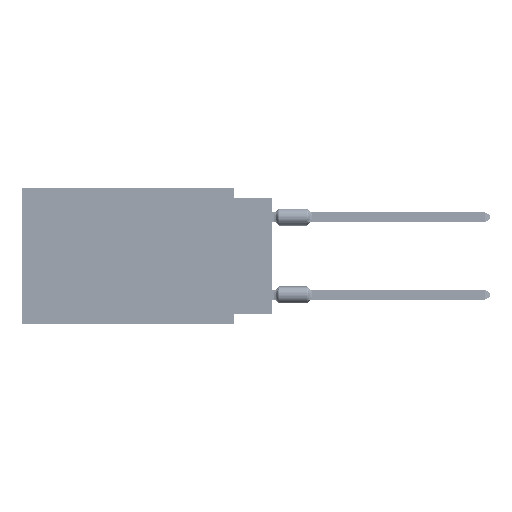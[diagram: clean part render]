
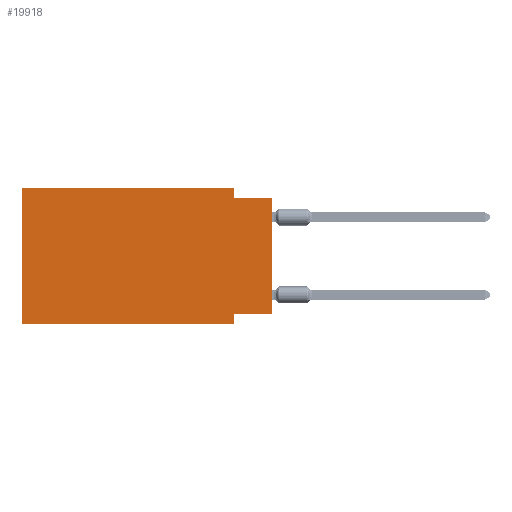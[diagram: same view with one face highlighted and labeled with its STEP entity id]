
A CAD part, left-side view. The second image highlights one B-rep face of the part: STEP entity #19918.
In plain terms, the highlighted planar face has unit normal (-1, 0, 0).
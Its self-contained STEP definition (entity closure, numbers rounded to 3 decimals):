
#172 = VERTEX_POINT ( 'NONE', #66391 ) ;
#1772 = LINE ( 'NONE', #67572, #3884 ) ;
#1815 = LINE ( 'NONE', #30420, #67050 ) ;
#2277 = DIRECTION ( 'NONE',  ( 0., 0., -1. ) ) ;
#2451 = EDGE_CURVE ( 'NONE', #49200, #65227, #50712, .T. ) ;
#3884 = VECTOR ( 'NONE', #35397, 1000. ) ;
#5882 = EDGE_CURVE ( 'NONE', #38103, #64522, #67398, .T. ) ;
#8389 = CARTESIAN_POINT ( 'NONE',  ( 0., 16.383, 0. ) ) ;
#10590 = DIRECTION ( 'NONE',  ( 0., -1., 0. ) ) ;
#10995 = DIRECTION ( 'NONE',  ( 0., 0., -1. ) ) ;
#12068 = EDGE_CURVE ( 'NONE', #49200, #19181, #1815, .T. ) ;
#12391 = FACE_OUTER_BOUND ( 'NONE', #24524, .T. ) ;
#12563 = CARTESIAN_POINT ( 'NONE',  ( 0., 2.54, -8.255 ) ) ;
#14311 = DIRECTION ( 'NONE',  ( 0., 1., 0. ) ) ;
#15615 = CARTESIAN_POINT ( 'NONE',  ( 0., 16.383, -8.89 ) ) ;
#16033 = AXIS2_PLACEMENT_3D ( 'NONE', #54968, #59996, #10995 ) ;
#16407 = CARTESIAN_POINT ( 'NONE',  ( 0., 0., -0.635 ) ) ;
#17709 = VECTOR ( 'NONE', #62150, 1000. ) ;
#18335 = DIRECTION ( 'NONE',  ( 0., 0., 1. ) ) ;
#18380 = CARTESIAN_POINT ( 'NONE',  ( 0., 2.54, 0. ) ) ;
#19181 = VERTEX_POINT ( 'NONE', #12563 ) ;
#19918 = ADVANCED_FACE ( 'NONE', ( #12391 ), #49604, .F. ) ;
#24398 = VERTEX_POINT ( 'NONE', #56808 ) ;
#24524 = EDGE_LOOP ( 'NONE', ( #34613, #55783, #64767, #27167, #53385, #25522, #66398, #43980 ) ) ;
#25398 = CARTESIAN_POINT ( 'NONE',  ( 0., 2.54, -8.89 ) ) ;
#25522 = ORIENTED_EDGE ( 'NONE', *, *, #68546, .T. ) ;
#27102 = EDGE_CURVE ( 'NONE', #172, #24398, #61634, .T. ) ;
#27167 = ORIENTED_EDGE ( 'NONE', *, *, #41906, .F. ) ;
#30194 = CARTESIAN_POINT ( 'NONE',  ( 0., 0., -0.635 ) ) ;
#30420 = CARTESIAN_POINT ( 'NONE',  ( 0., 0., -8.255 ) ) ;
#33171 = VECTOR ( 'NONE', #10590, 1000. ) ;
#33748 = CARTESIAN_POINT ( 'NONE',  ( 0., 2.54, -0.635 ) ) ;
#33891 = EDGE_CURVE ( 'NONE', #19181, #54962, #1772, .T. ) ;
#34609 = CARTESIAN_POINT ( 'NONE',  ( 0., 0., 0. ) ) ;
#34613 = ORIENTED_EDGE ( 'NONE', *, *, #2451, .T. ) ;
#35397 = DIRECTION ( 'NONE',  ( 0., 0., -1. ) ) ;
#35580 = LINE ( 'NONE', #8389, #62448 ) ;
#38103 = VERTEX_POINT ( 'NONE', #56673 ) ;
#40477 = VECTOR ( 'NONE', #57369, 1000. ) ;
#41270 = LINE ( 'NONE', #30194, #40477 ) ;
#41906 = EDGE_CURVE ( 'NONE', #24398, #38103, #35580, .T. ) ;
#43980 = ORIENTED_EDGE ( 'NONE', *, *, #12068, .F. ) ;
#44009 = VECTOR ( 'NONE', #2277, 1000. ) ;
#49200 = VERTEX_POINT ( 'NONE', #57150 ) ;
#49604 = PLANE ( 'NONE',  #16033 ) ;
#50712 = LINE ( 'NONE', #34609, #17709 ) ;
#50892 = CARTESIAN_POINT ( 'NONE',  ( 0., 16.383, 0. ) ) ;
#51060 = EDGE_CURVE ( 'NONE', #64522, #65227, #41270, .T. ) ;
#52050 = DIRECTION ( 'NONE',  ( 0., -1., 0. ) ) ;
#53385 = ORIENTED_EDGE ( 'NONE', *, *, #27102, .F. ) ;
#54962 = VERTEX_POINT ( 'NONE', #25398 ) ;
#54968 = CARTESIAN_POINT ( 'NONE',  ( 0., 16.383, 0. ) ) ;
#55783 = ORIENTED_EDGE ( 'NONE', *, *, #51060, .F. ) ;
#56673 = CARTESIAN_POINT ( 'NONE',  ( 0., 2.54, 0. ) ) ;
#56808 = CARTESIAN_POINT ( 'NONE',  ( 0., 16.383, 0. ) ) ;
#57150 = CARTESIAN_POINT ( 'NONE',  ( 0., 0., -8.255 ) ) ;
#57369 = DIRECTION ( 'NONE',  ( 0., -1., 0. ) ) ;
#57708 = VECTOR ( 'NONE', #18335, 1000. ) ;
#59996 = DIRECTION ( 'NONE',  ( 1., 0., 0. ) ) ;
#61634 = LINE ( 'NONE', #50892, #57708 ) ;
#62150 = DIRECTION ( 'NONE',  ( 0., 0., 1. ) ) ;
#62448 = VECTOR ( 'NONE', #52050, 1000. ) ;
#64522 = VERTEX_POINT ( 'NONE', #33748 ) ;
#64767 = ORIENTED_EDGE ( 'NONE', *, *, #5882, .F. ) ;
#65227 = VERTEX_POINT ( 'NONE', #16407 ) ;
#65674 = LINE ( 'NONE', #15615, #33171 ) ;
#66391 = CARTESIAN_POINT ( 'NONE',  ( 0., 16.383, -8.89 ) ) ;
#66398 = ORIENTED_EDGE ( 'NONE', *, *, #33891, .F. ) ;
#67050 = VECTOR ( 'NONE', #14311, 1000. ) ;
#67398 = LINE ( 'NONE', #18380, #44009 ) ;
#67572 = CARTESIAN_POINT ( 'NONE',  ( 0., 2.54, -8.89 ) ) ;
#68546 = EDGE_CURVE ( 'NONE', #172, #54962, #65674, .T. ) ;
